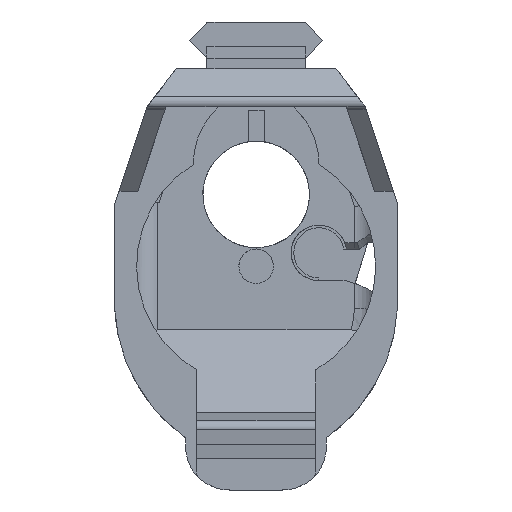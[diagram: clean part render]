
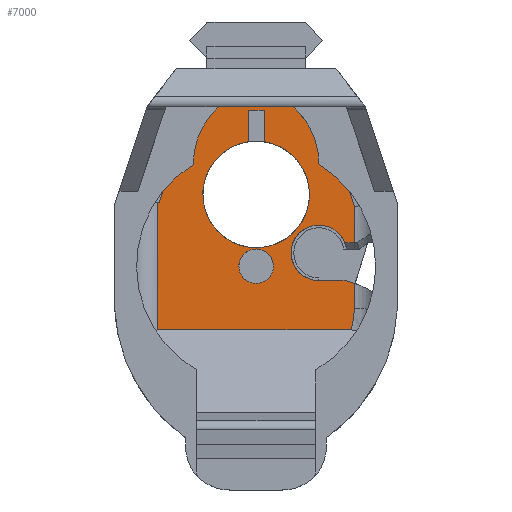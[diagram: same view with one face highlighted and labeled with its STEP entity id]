
A CAD part, front view. The second image highlights one B-rep face of the part: STEP entity #7000.
In plain terms, the highlighted planar face has unit normal (0, -1, 0).
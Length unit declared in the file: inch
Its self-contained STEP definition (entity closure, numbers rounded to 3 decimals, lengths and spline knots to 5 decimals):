
#43=FACE_BOUND('',#1032,.T.);
#44=FACE_BOUND('',#1033,.T.);
#305=PLANE('',#7519);
#658=FACE_OUTER_BOUND('',#1031,.T.);
#1031=EDGE_LOOP('',(#5862,#5863,#5864,#5865,#5866,#5867,#5868,#5869,#5870,
#5871,#5872,#5873,#5874,#5875,#5876,#5877));
#1032=EDGE_LOOP('',(#5878,#5879));
#1033=EDGE_LOOP('',(#5880,#5881,#5882,#5883,#5884));
#1357=LINE('',#10091,#2201);
#1403=LINE('',#10202,#2247);
#1408=LINE('',#10217,#2252);
#1419=LINE('',#10253,#2263);
#1423=LINE('',#10262,#2267);
#1453=LINE('',#10358,#2297);
#1564=LINE('',#10661,#2408);
#1620=LINE('',#10832,#2464);
#1627=LINE('',#10860,#2471);
#1643=LINE('',#10953,#2487);
#1716=LINE('',#11162,#2560);
#1720=LINE('',#11191,#2564);
#1721=LINE('',#11194,#2565);
#1722=LINE('',#11197,#2566);
#1723=LINE('',#11199,#2567);
#1724=LINE('',#11202,#2568);
#1725=LINE('',#11203,#2569);
#2201=VECTOR('',#8099,0.3937);
#2247=VECTOR('',#8177,0.3937);
#2252=VECTOR('',#8186,0.3937);
#2263=VECTOR('',#8217,0.3937);
#2267=VECTOR('',#8225,0.3937);
#2297=VECTOR('',#8279,0.3937);
#2408=VECTOR('',#8514,0.3937);
#2464=VECTOR('',#8634,0.3937);
#2471=VECTOR('',#8653,0.3937);
#2487=VECTOR('',#8679,0.3937);
#2560=VECTOR('',#8888,0.3937);
#2564=VECTOR('',#8900,0.3937);
#2565=VECTOR('',#8903,0.3937);
#2566=VECTOR('',#8908,0.3937);
#2567=VECTOR('',#8909,0.3937);
#2568=VECTOR('',#8912,0.3937);
#2569=VECTOR('',#8913,0.3937);
#2929=CIRCLE('',#7299,0.33465);
#2930=CIRCLE('',#7300,0.33465);
#2947=CIRCLE('',#7420,0.17421);
#2954=CIRCLE('',#7451,0.10827);
#2955=CIRCLE('',#7452,0.10827);
#2961=CIRCLE('',#7520,0.78536);
#3127=VERTEX_POINT('',#10088);
#3128=VERTEX_POINT('',#10090);
#3129=VERTEX_POINT('',#10094);
#3130=VERTEX_POINT('',#10097);
#3165=VERTEX_POINT('',#10199);
#3166=VERTEX_POINT('',#10201);
#3171=VERTEX_POINT('',#10215);
#3185=VERTEX_POINT('',#10250);
#3186=VERTEX_POINT('',#10252);
#3189=VERTEX_POINT('',#10260);
#3217=VERTEX_POINT('',#10356);
#3314=VERTEX_POINT('',#10660);
#3338=VERTEX_POINT('',#10733);
#3355=VERTEX_POINT('',#10829);
#3356=VERTEX_POINT('',#10831);
#3365=VERTEX_POINT('',#10859);
#3377=VERTEX_POINT('',#10951);
#3383=VERTEX_POINT('',#10970);
#3384=VERTEX_POINT('',#10971);
#3423=VERTEX_POINT('',#11189);
#3424=VERTEX_POINT('',#11193);
#3425=VERTEX_POINT('',#11198);
#3426=VERTEX_POINT('',#11201);
#3852=EDGE_CURVE('',#3128,#3127,#1357,.T.);
#3855=EDGE_CURVE('',#3127,#3129,#2929,.T.);
#3857=EDGE_CURVE('',#3129,#3130,#2930,.T.);
#3905=EDGE_CURVE('',#3165,#3166,#1403,.T.);
#3912=EDGE_CURVE('',#3165,#3171,#1408,.T.);
#3929=EDGE_CURVE('',#3185,#3186,#1419,.T.);
#3934=EDGE_CURVE('',#3185,#3189,#1423,.T.);
#3970=EDGE_CURVE('',#3189,#3217,#1453,.T.);
#4107=EDGE_CURVE('',#3314,#3186,#1564,.T.);
#4146=EDGE_CURVE('',#3171,#3338,#2947,.T.);
#4177=EDGE_CURVE('',#3355,#3356,#1620,.T.);
#4189=EDGE_CURVE('',#3166,#3365,#1627,.T.);
#4210=EDGE_CURVE('',#3377,#3338,#1643,.T.);
#4218=EDGE_CURVE('',#3383,#3384,#2954,.T.);
#4219=EDGE_CURVE('',#3384,#3383,#2955,.T.);
#4309=EDGE_CURVE('',#3356,#3217,#1716,.T.);
#4316=EDGE_CURVE('',#3423,#3355,#1720,.T.);
#4317=EDGE_CURVE('',#3314,#3424,#1721,.T.);
#4319=EDGE_CURVE('',#3424,#3377,#1722,.T.);
#4320=EDGE_CURVE('',#3423,#3425,#1723,.T.);
#4321=EDGE_CURVE('',#3365,#3425,#2961,.T.);
#4322=EDGE_CURVE('',#3130,#3426,#1724,.T.);
#4323=EDGE_CURVE('',#3426,#3128,#1725,.T.);
#5862=ORIENTED_EDGE('',*,*,#4210,.F.);
#5863=ORIENTED_EDGE('',*,*,#4319,.F.);
#5864=ORIENTED_EDGE('',*,*,#4317,.F.);
#5865=ORIENTED_EDGE('',*,*,#4107,.T.);
#5866=ORIENTED_EDGE('',*,*,#3929,.F.);
#5867=ORIENTED_EDGE('',*,*,#3934,.T.);
#5868=ORIENTED_EDGE('',*,*,#3970,.T.);
#5869=ORIENTED_EDGE('',*,*,#4309,.F.);
#5870=ORIENTED_EDGE('',*,*,#4177,.F.);
#5871=ORIENTED_EDGE('',*,*,#4316,.F.);
#5872=ORIENTED_EDGE('',*,*,#4320,.T.);
#5873=ORIENTED_EDGE('',*,*,#4321,.F.);
#5874=ORIENTED_EDGE('',*,*,#4189,.F.);
#5875=ORIENTED_EDGE('',*,*,#3905,.F.);
#5876=ORIENTED_EDGE('',*,*,#3912,.T.);
#5877=ORIENTED_EDGE('',*,*,#4146,.T.);
#5878=ORIENTED_EDGE('',*,*,#4218,.T.);
#5879=ORIENTED_EDGE('',*,*,#4219,.T.);
#5880=ORIENTED_EDGE('',*,*,#3852,.T.);
#5881=ORIENTED_EDGE('',*,*,#3855,.T.);
#5882=ORIENTED_EDGE('',*,*,#3857,.T.);
#5883=ORIENTED_EDGE('',*,*,#4322,.T.);
#5884=ORIENTED_EDGE('',*,*,#4323,.T.);
#7000=ADVANCED_FACE('',(#658,#43,#44),#305,.T.);
#7299=AXIS2_PLACEMENT_3D('',#10096,#8104,#8105);
#7300=AXIS2_PLACEMENT_3D('',#10099,#8107,#8108);
#7420=AXIS2_PLACEMENT_3D('',#10735,#8582,#8583);
#7451=AXIS2_PLACEMENT_3D('',#10972,#8697,#8698);
#7452=AXIS2_PLACEMENT_3D('',#10973,#8699,#8700);
#7519=AXIS2_PLACEMENT_3D('',#11196,#8906,#8907);
#7520=AXIS2_PLACEMENT_3D('',#11200,#8910,#8911);
#8099=DIRECTION('',(0.,0.,-1.));
#8104=DIRECTION('center_axis',(0.,1.,0.));
#8105=DIRECTION('ref_axis',(-1.,0.,0.));
#8107=DIRECTION('center_axis',(0.,1.,0.));
#8108=DIRECTION('ref_axis',(-1.,0.,0.));
#8177=DIRECTION('',(0.954,0.,-0.301));
#8186=DIRECTION('',(-1.,0.,0.));
#8217=DIRECTION('',(1.,0.,-0.002));
#8225=DIRECTION('',(0.,0.,-1.));
#8279=DIRECTION('',(-1.,0.,0.));
#8514=DIRECTION('',(0.002,0.,1.));
#8582=DIRECTION('center_axis',(0.,1.,0.));
#8583=DIRECTION('ref_axis',(1.,0.,0.));
#8634=DIRECTION('',(1.,0.,0.));
#8653=DIRECTION('',(0.,0.,-1.));
#8679=DIRECTION('',(-1.,0.,0.));
#8697=DIRECTION('center_axis',(0.,1.,0.));
#8698=DIRECTION('ref_axis',(1.,0.,0.));
#8699=DIRECTION('center_axis',(0.,1.,0.));
#8700=DIRECTION('ref_axis',(1.,0.,0.));
#8888=DIRECTION('',(0.316,0.,0.949));
#8900=DIRECTION('',(0.,0.,1.));
#8903=DIRECTION('',(0.316,0.,-0.949));
#8906=DIRECTION('center_axis',(0.,-1.,0.));
#8907=DIRECTION('ref_axis',(0.,0.,-1.));
#8908=DIRECTION('',(0.,0.,-1.));
#8909=DIRECTION('',(1.,0.,0.));
#8910=DIRECTION('center_axis',(0.,1.,0.));
#8911=DIRECTION('ref_axis',(0.992,0.,-0.128));
#8912=DIRECTION('',(0.,0.,1.));
#8913=DIRECTION('',(1.,0.,0.));
#10088=CARTESIAN_POINT('',(0.05072,2.56,0.78078));
#10090=CARTESIAN_POINT('',(0.05072,2.56,0.97719));
#10091=CARTESIAN_POINT('',(0.05072,2.56,0.54014));
#10094=CARTESIAN_POINT('',(0.33465,2.56,0.45));
#10096=CARTESIAN_POINT('Origin',(0.,2.56,0.45));
#10097=CARTESIAN_POINT('',(-0.0477,2.56,0.78123));
#10099=CARTESIAN_POINT('Origin',(0.,2.56,0.45));
#10199=CARTESIAN_POINT('',(0.55783,2.56,-0.08921));
#10201=CARTESIAN_POINT('',(0.61679,2.56,-0.1078));
#10202=CARTESIAN_POINT('',(0.05278,2.56,0.07004));
#10215=CARTESIAN_POINT('',(0.41433,2.56,-0.08921));
#10217=CARTESIAN_POINT('',(0.10264,2.56,-0.08921));
#10250=CARTESIAN_POINT('',(0.5,2.56,1.0001));
#10252=CARTESIAN_POINT('',(0.56627,2.56,0.99997));
#10253=CARTESIAN_POINT('',(0.5,2.56,1.0001));
#10260=CARTESIAN_POINT('',(0.5,2.56,0.99982));
#10262=CARTESIAN_POINT('',(0.5,2.56,0.64988));
#10356=CARTESIAN_POINT('',(-0.40817,2.56,0.99982));
#10358=CARTESIAN_POINT('',(-0.5,2.56,0.99982));
#10660=CARTESIAN_POINT('',(0.56534,2.56,0.52831));
#10661=CARTESIAN_POINT('',(0.56627,2.56,0.99987));
#10733=CARTESIAN_POINT('',(0.55575,2.56,0.14773));
#10735=CARTESIAN_POINT('Origin',(0.3937,2.56,0.08378));
#10829=CARTESIAN_POINT('',(-0.61864,2.56,0.39831));
#10831=CARTESIAN_POINT('',(-0.60868,2.56,0.39831));
#10832=CARTESIAN_POINT('',(-0.79245,2.56,0.39831));
#10859=CARTESIAN_POINT('',(0.61679,2.56,-0.26638));
#10860=CARTESIAN_POINT('',(0.61679,2.56,0.01448));
#10951=CARTESIAN_POINT('',(0.61679,2.56,0.14773));
#10953=CARTESIAN_POINT('',(0.03313,2.56,0.14773));
#10970=CARTESIAN_POINT('',(-0.05174,2.56,0.0951));
#10971=CARTESIAN_POINT('',(-0.10827,2.56,0.));
#10972=CARTESIAN_POINT('Origin',(0.,2.56,0.));
#10973=CARTESIAN_POINT('Origin',(0.,2.56,0.));
#11162=CARTESIAN_POINT('',(-0.6259,2.56,0.34662));
#11189=CARTESIAN_POINT('',(-0.61864,2.56,-0.4));
#11191=CARTESIAN_POINT('',(-0.61864,2.56,0.34912));
#11193=CARTESIAN_POINT('',(0.61679,2.56,0.37396));
#11194=CARTESIAN_POINT('',(0.47564,2.56,0.79741));
#11196=CARTESIAN_POINT('Origin',(-0.5,2.56,0.29994));
#11197=CARTESIAN_POINT('',(0.61679,2.56,0.01448));
#11198=CARTESIAN_POINT('',(0.59654,2.56,-0.4));
#11199=CARTESIAN_POINT('',(0.37309,2.56,-0.4));
#11200=CARTESIAN_POINT('Origin',(-0.16695,2.56,-0.21593));
#11201=CARTESIAN_POINT('',(-0.0477,2.56,0.97719));
#11202=CARTESIAN_POINT('',(-0.0477,2.56,0.54014));
#11203=CARTESIAN_POINT('',(-0.22464,2.56,0.97719));
